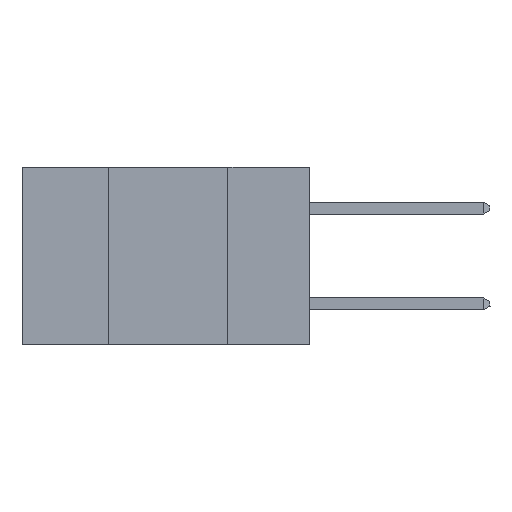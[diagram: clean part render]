
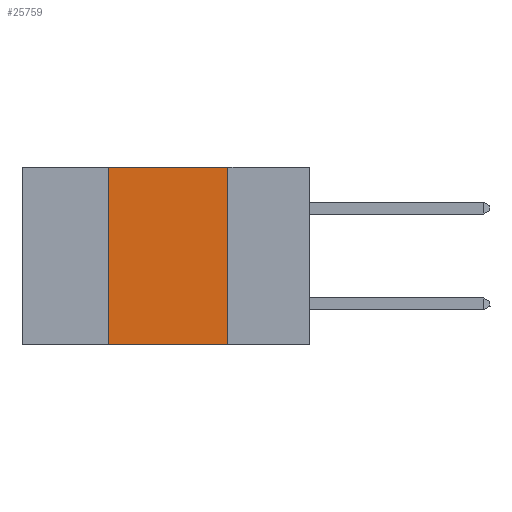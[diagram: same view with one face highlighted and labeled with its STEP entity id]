
A CAD part, left-side view. The second image highlights one B-rep face of the part: STEP entity #25759.
In plain terms, the highlighted planar face has unit normal (-1, 0, 0).
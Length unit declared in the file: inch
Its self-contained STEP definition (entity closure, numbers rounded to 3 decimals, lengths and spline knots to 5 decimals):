
#282 = DIRECTION ( 'NONE',  ( 0., 0., -1. ) ) ;
#1863 = CARTESIAN_POINT ( 'NONE',  ( 0., 0.6, 0. ) ) ;
#3928 = DIRECTION ( 'NONE',  ( 0., 0., -1. ) ) ;
#4370 = CARTESIAN_POINT ( 'NONE',  ( 0., 0.17, 0. ) ) ;
#4733 = CARTESIAN_POINT ( 'NONE',  ( 0., 0.17, -0.37 ) ) ;
#5892 = PLANE ( 'NONE',  #10256 ) ;
#6275 = EDGE_LOOP ( 'NONE', ( #19018, #22137, #21505, #20570 ) ) ;
#7681 = VECTOR ( 'NONE', #13738, 39.37008 ) ;
#7993 = DIRECTION ( 'NONE',  ( 0., -1., 0. ) ) ;
#9719 = CARTESIAN_POINT ( 'NONE',  ( 0., 0.17, 0. ) ) ;
#10256 = AXIS2_PLACEMENT_3D ( 'NONE', #1863, #16000, #3928 ) ;
#10990 = LINE ( 'NONE', #4370, #21049 ) ;
#11266 = CARTESIAN_POINT ( 'NONE',  ( 0., 0.6, -0.37 ) ) ;
#13031 = LINE ( 'NONE', #25539, #7681 ) ;
#13146 = LINE ( 'NONE', #11266, #18462 ) ;
#13738 = DIRECTION ( 'NONE',  ( 0., 0., 1. ) ) ;
#14179 = FACE_OUTER_BOUND ( 'NONE', #6275, .T. ) ;
#15125 = VERTEX_POINT ( 'NONE', #25612 ) ;
#15416 = CARTESIAN_POINT ( 'NONE',  ( 0., 0.42, -0.37 ) ) ;
#16000 = DIRECTION ( 'NONE',  ( 1., 0., 0. ) ) ;
#16268 = VECTOR ( 'NONE', #7993, 39.37008 ) ;
#17681 = VERTEX_POINT ( 'NONE', #9719 ) ;
#18462 = VECTOR ( 'NONE', #21281, 39.37008 ) ;
#18544 = EDGE_CURVE ( 'NONE', #23123, #19683, #13146, .T. ) ;
#19018 = ORIENTED_EDGE ( 'NONE', *, *, #25919, .F. ) ;
#19683 = VERTEX_POINT ( 'NONE', #4733 ) ;
#20030 = CARTESIAN_POINT ( 'NONE',  ( 0., 0.6, 0. ) ) ;
#20570 = ORIENTED_EDGE ( 'NONE', *, *, #18544, .T. ) ;
#21049 = VECTOR ( 'NONE', #282, 39.37008 ) ;
#21281 = DIRECTION ( 'NONE',  ( 0., -1., 0. ) ) ;
#21505 = ORIENTED_EDGE ( 'NONE', *, *, #23818, .F. ) ;
#22047 = EDGE_CURVE ( 'NONE', #15125, #17681, #22201, .T. ) ;
#22137 = ORIENTED_EDGE ( 'NONE', *, *, #22047, .F. ) ;
#22201 = LINE ( 'NONE', #20030, #16268 ) ;
#23123 = VERTEX_POINT ( 'NONE', #15416 ) ;
#23818 = EDGE_CURVE ( 'NONE', #23123, #15125, #13031, .T. ) ;
#25539 = CARTESIAN_POINT ( 'NONE',  ( 0., 0.42, 0. ) ) ;
#25612 = CARTESIAN_POINT ( 'NONE',  ( 0., 0.42, 0. ) ) ;
#25759 = ADVANCED_FACE ( 'NONE', ( #14179 ), #5892, .F. ) ;
#25919 = EDGE_CURVE ( 'NONE', #17681, #19683, #10990, .T. ) ;
